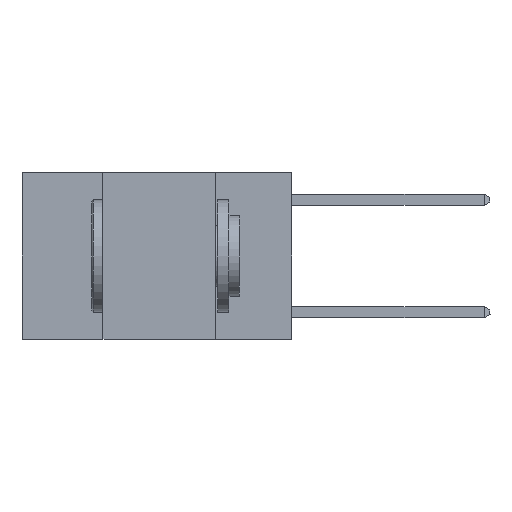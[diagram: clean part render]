
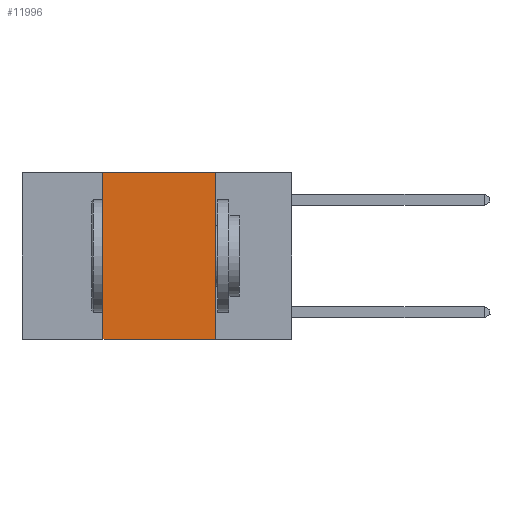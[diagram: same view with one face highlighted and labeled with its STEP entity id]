
A CAD part, left-side view. The second image highlights one B-rep face of the part: STEP entity #11996.
In plain terms, the highlighted planar face has unit normal (-1, 0, 0).
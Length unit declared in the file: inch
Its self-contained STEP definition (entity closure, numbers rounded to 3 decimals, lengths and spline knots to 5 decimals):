
#662 = VECTOR ( 'NONE', #3082, 39.37008 ) ;
#907 = LINE ( 'NONE', #1199, #8337 ) ;
#1060 = DIRECTION ( 'NONE',  ( 0., -1., 0. ) ) ;
#1199 = CARTESIAN_POINT ( 'NONE',  ( 0., 0.42, 0. ) ) ;
#1326 = VECTOR ( 'NONE', #1060, 39.37008 ) ;
#1623 = LINE ( 'NONE', #4832, #1326 ) ;
#1892 = CARTESIAN_POINT ( 'NONE',  ( 0., 0.6, 0. ) ) ;
#1897 = EDGE_LOOP ( 'NONE', ( #2022, #2064, #2135, #2232 ) ) ;
#2022 = ORIENTED_EDGE ( 'NONE', *, *, #6830, .F. ) ;
#2064 = ORIENTED_EDGE ( 'NONE', *, *, #4243, .F. ) ;
#2135 = ORIENTED_EDGE ( 'NONE', *, *, #6791, .F. ) ;
#2232 = ORIENTED_EDGE ( 'NONE', *, *, #8574, .T. ) ;
#3082 = DIRECTION ( 'NONE',  ( 0., -1., 0. ) ) ;
#4243 = EDGE_CURVE ( 'NONE', #4516, #12365, #1623, .T. ) ;
#4286 = CARTESIAN_POINT ( 'NONE',  ( 0., 0.42, -0.37 ) ) ;
#4516 = VERTEX_POINT ( 'NONE', #8808 ) ;
#4832 = CARTESIAN_POINT ( 'NONE',  ( 0., 0.6, 0. ) ) ;
#4990 = FACE_OUTER_BOUND ( 'NONE', #1897, .T. ) ;
#5366 = VERTEX_POINT ( 'NONE', #4286 ) ;
#5410 = AXIS2_PLACEMENT_3D ( 'NONE', #1892, #11513, #5693 ) ;
#5693 = DIRECTION ( 'NONE',  ( 0., 0., -1. ) ) ;
#5703 = LINE ( 'NONE', #7981, #662 ) ;
#6791 = EDGE_CURVE ( 'NONE', #5366, #4516, #907, .T. ) ;
#6830 = EDGE_CURVE ( 'NONE', #12365, #10939, #7012, .T. ) ;
#7012 = LINE ( 'NONE', #9991, #11843 ) ;
#7025 = DIRECTION ( 'NONE',  ( 0., 0., -1. ) ) ;
#7981 = CARTESIAN_POINT ( 'NONE',  ( 0., 0.6, -0.37 ) ) ;
#8337 = VECTOR ( 'NONE', #8916, 39.37008 ) ;
#8574 = EDGE_CURVE ( 'NONE', #5366, #10939, #5703, .T. ) ;
#8808 = CARTESIAN_POINT ( 'NONE',  ( 0., 0.42, 0. ) ) ;
#8916 = DIRECTION ( 'NONE',  ( 0., 0., 1. ) ) ;
#9991 = CARTESIAN_POINT ( 'NONE',  ( 0., 0.17, 0. ) ) ;
#10627 = PLANE ( 'NONE',  #5410 ) ;
#10939 = VERTEX_POINT ( 'NONE', #11521 ) ;
#10992 = CARTESIAN_POINT ( 'NONE',  ( 0., 0.17, 0. ) ) ;
#11513 = DIRECTION ( 'NONE',  ( 1., 0., 0. ) ) ;
#11521 = CARTESIAN_POINT ( 'NONE',  ( 0., 0.17, -0.37 ) ) ;
#11843 = VECTOR ( 'NONE', #7025, 39.37008 ) ;
#11996 = ADVANCED_FACE ( 'NONE', ( #4990 ), #10627, .F. ) ;
#12365 = VERTEX_POINT ( 'NONE', #10992 ) ;
